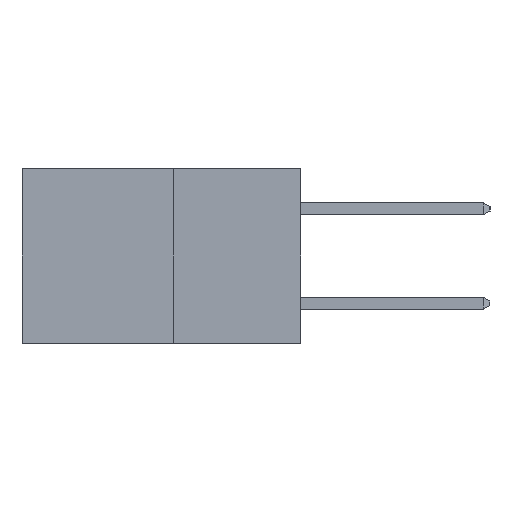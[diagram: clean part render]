
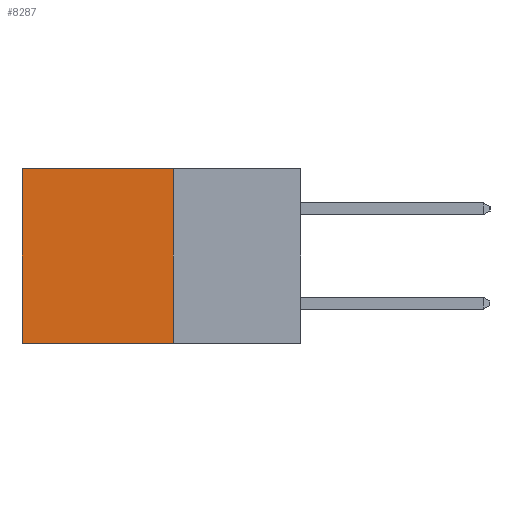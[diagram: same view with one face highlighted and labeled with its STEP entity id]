
A CAD part, left-side view. The second image highlights one B-rep face of the part: STEP entity #8287.
In plain terms, the highlighted planar face has unit normal (-1, 0, 0).
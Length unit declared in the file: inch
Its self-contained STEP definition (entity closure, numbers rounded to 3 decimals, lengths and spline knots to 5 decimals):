
#336 = EDGE_CURVE ( 'NONE', #12090, #4249, #10265, .T. ) ;
#654 = CARTESIAN_POINT ( 'NONE',  ( 0.277, 0.27, 0. ) ) ;
#705 = EDGE_CURVE ( 'NONE', #1213, #12090, #4073, .T. ) ;
#1060 = VECTOR ( 'NONE', #2301, 39.37008 ) ;
#1213 = VERTEX_POINT ( 'NONE', #4205 ) ;
#2038 = ORIENTED_EDGE ( 'NONE', *, *, #5914, .F. ) ;
#2301 = DIRECTION ( 'NONE',  ( 0., 1., 0. ) ) ;
#2337 = VERTEX_POINT ( 'NONE', #8440 ) ;
#2340 = VECTOR ( 'NONE', #12041, 39.37008 ) ;
#3079 = CARTESIAN_POINT ( 'NONE',  ( 0.277, 0.59, -0.37 ) ) ;
#3321 = CARTESIAN_POINT ( 'NONE',  ( 0.277, 0.27, -0.37 ) ) ;
#3376 = CARTESIAN_POINT ( 'NONE',  ( 0.277, 0.59, -0.37 ) ) ;
#4073 = LINE ( 'NONE', #654, #2340 ) ;
#4205 = CARTESIAN_POINT ( 'NONE',  ( 0.277, 0.27, 0. ) ) ;
#4249 = VERTEX_POINT ( 'NONE', #3079 ) ;
#4794 = EDGE_LOOP ( 'NONE', ( #9164, #11536, #2038, #7036 ) ) ;
#4985 = PLANE ( 'NONE',  #7190 ) ;
#5740 = VECTOR ( 'NONE', #10966, 39.37008 ) ;
#5914 = EDGE_CURVE ( 'NONE', #1213, #2337, #8697, .T. ) ;
#6090 = CARTESIAN_POINT ( 'NONE',  ( 0.277, 0.59, 0. ) ) ;
#6557 = DIRECTION ( 'NONE',  ( 0., 0., -1. ) ) ;
#6803 = DIRECTION ( 'NONE',  ( 0., 0., -1. ) ) ;
#7036 = ORIENTED_EDGE ( 'NONE', *, *, #705, .T. ) ;
#7190 = AXIS2_PLACEMENT_3D ( 'NONE', #11277, #12131, #6803 ) ;
#7248 = FACE_OUTER_BOUND ( 'NONE', #4794, .T. ) ;
#8287 = ADVANCED_FACE ( 'NONE', ( #7248 ), #4985, .F. ) ;
#8440 = CARTESIAN_POINT ( 'NONE',  ( 0.277, 0.27, -0.37 ) ) ;
#8697 = LINE ( 'NONE', #11031, #10788 ) ;
#9164 = ORIENTED_EDGE ( 'NONE', *, *, #336, .T. ) ;
#9378 = EDGE_CURVE ( 'NONE', #2337, #4249, #11024, .T. ) ;
#10265 = LINE ( 'NONE', #3376, #5740 ) ;
#10788 = VECTOR ( 'NONE', #6557, 39.37008 ) ;
#10966 = DIRECTION ( 'NONE',  ( 0., 0., -1. ) ) ;
#11024 = LINE ( 'NONE', #3321, #1060 ) ;
#11031 = CARTESIAN_POINT ( 'NONE',  ( 0.277, 0.27, -0.37 ) ) ;
#11277 = CARTESIAN_POINT ( 'NONE',  ( 0.277, 0.27, -0.37 ) ) ;
#11536 = ORIENTED_EDGE ( 'NONE', *, *, #9378, .F. ) ;
#12041 = DIRECTION ( 'NONE',  ( 0., 1., 0. ) ) ;
#12090 = VERTEX_POINT ( 'NONE', #6090 ) ;
#12131 = DIRECTION ( 'NONE',  ( 1., 0., 0. ) ) ;
